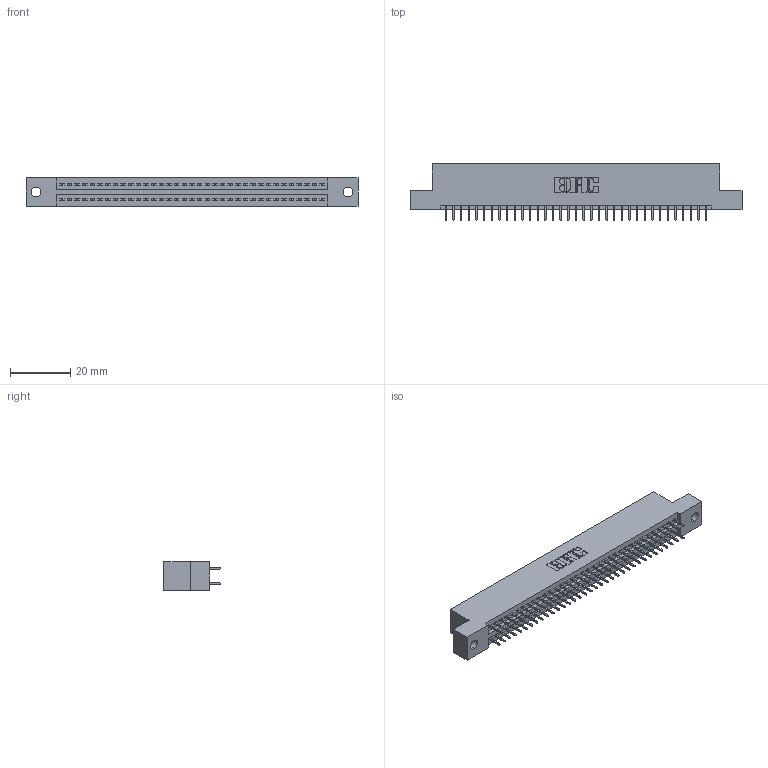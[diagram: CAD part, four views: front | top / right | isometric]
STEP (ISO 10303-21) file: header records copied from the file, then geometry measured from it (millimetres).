
FILE_DESCRIPTION (( 'STEP AP203' ), '1' );
FILE_NAME ('845-070-525-202.STEP', '2020-09-23T21:40:03', ( '' ), ( '' ), 'SwSTEP 2.0', 'SolidWorks 2020', '' );
FILE_SCHEMA (( 'CONFIG_CONTROL_DESIGN' ));
Length unit declared in the file: inch
Products named in the file (3): 845-070-525-202; 845 Part_Flush Mounting Lugs - 0.128 Dia; 345-292-001_345-293-125
Assembly tree (71 placements, depth 2):
  845-070-525-202
    845 Part_Flush Mounting Lugs - 0.128 Dia
    345-292-001_345-293-125  x70
Bounding box: 110.11 x 18.72 x 9.4 mm (x, y, z)
Volume: 10479.2 mm3; surface area: 14734.5 mm2
Topology: 71 solids, 71 shells, 3906 faces, 11051 edges, 7086 vertices
Faces by surface type: plane 2810, cylinder 1096
Entity records: 28481 total; most frequent: CARTESIAN_POINT 4780, ORIENTED_EDGE 4714, DIRECTION 4225, EDGE_CURVE 2357, LINE 2089, VECTOR 2089, VERTEX_POINT 1566, AXIS2_PLACEMENT_3D 1068
